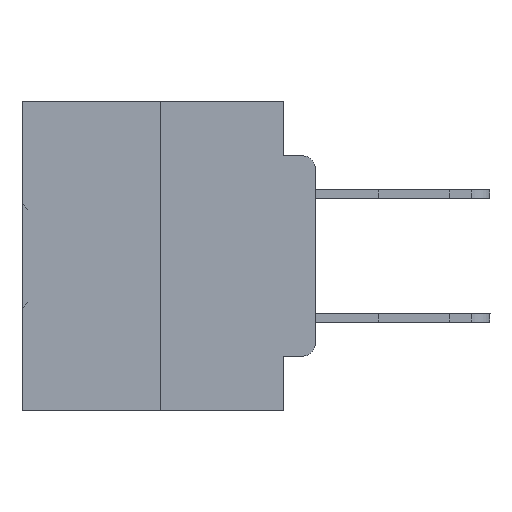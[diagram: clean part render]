
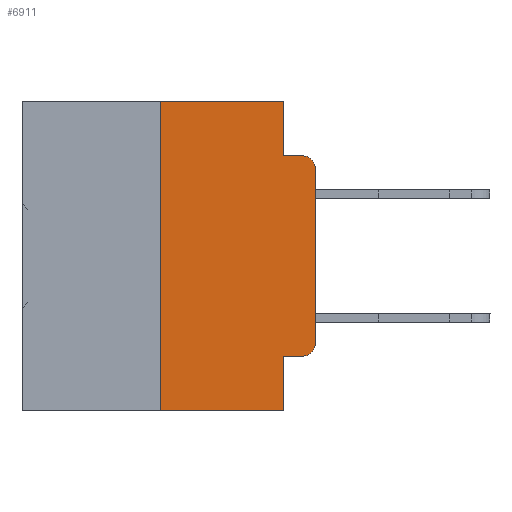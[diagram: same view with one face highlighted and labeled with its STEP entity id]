
A CAD part, left-side view. The second image highlights one B-rep face of the part: STEP entity #6911.
In plain terms, the highlighted planar face has unit normal (-1, 0, 0).
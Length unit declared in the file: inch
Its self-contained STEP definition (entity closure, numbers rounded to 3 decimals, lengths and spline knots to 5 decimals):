
#1112 = EDGE_CURVE ( 'NONE', #8492, #10037, #37181, .T. ) ;
#1606 = DIRECTION ( 'NONE',  ( 0., -1., 0. ) ) ;
#2533 = VECTOR ( 'NONE', #21552, 39.37008 ) ;
#2599 = CARTESIAN_POINT ( 'NONE',  ( 0., 0.051, -0.0885 ) ) ;
#3186 = DIRECTION ( 'NONE',  ( 0., 0., -1. ) ) ;
#3960 = EDGE_LOOP ( 'NONE', ( #23107, #32588, #10582, #7675, #37081, #15077, #35755, #18304, #5383, #36278 ) ) ;
#5097 = LINE ( 'NONE', #10026, #2533 ) ;
#5383 = ORIENTED_EDGE ( 'NONE', *, *, #35285, .T. ) ;
#5484 = DIRECTION ( 'NONE',  ( 0., 0., -1. ) ) ;
#6058 = AXIS2_PLACEMENT_3D ( 'NONE', #34213, #8325, #31364 ) ;
#6208 = VECTOR ( 'NONE', #13456, 39.37008 ) ;
#6746 = AXIS2_PLACEMENT_3D ( 'NONE', #25912, #11363, #5484 ) ;
#6911 = ADVANCED_FACE ( 'NONE', ( #29285 ), #20406, .F. ) ;
#6920 = VERTEX_POINT ( 'NONE', #20225 ) ;
#6921 = EDGE_CURVE ( 'NONE', #34505, #21723, #31728, .T. ) ;
#7185 = VECTOR ( 'NONE', #19292, 39.37008 ) ;
#7336 = VECTOR ( 'NONE', #23421, 39.37008 ) ;
#7675 = ORIENTED_EDGE ( 'NONE', *, *, #26882, .F. ) ;
#7763 = CARTESIAN_POINT ( 'NONE',  ( 0., 0.051, 0. ) ) ;
#7807 = DIRECTION ( 'NONE',  ( 0., -1., 0. ) ) ;
#8325 = DIRECTION ( 'NONE',  ( 1., 0., 0. ) ) ;
#8492 = VERTEX_POINT ( 'NONE', #13720 ) ;
#8664 = CARTESIAN_POINT ( 'NONE',  ( 0., 0.051, -0.5 ) ) ;
#9150 = CIRCLE ( 'NONE', #6746, 0.02 ) ;
#10026 = CARTESIAN_POINT ( 'NONE',  ( 0., 0.473, -0.5 ) ) ;
#10037 = VERTEX_POINT ( 'NONE', #33516 ) ;
#10467 = CARTESIAN_POINT ( 'NONE',  ( 0., 0., -0.3915 ) ) ;
#10582 = ORIENTED_EDGE ( 'NONE', *, *, #1112, .F. ) ;
#11300 = VECTOR ( 'NONE', #1606, 39.37008 ) ;
#11363 = DIRECTION ( 'NONE',  ( -1., 0., 0. ) ) ;
#11385 = EDGE_CURVE ( 'NONE', #6920, #34505, #27099, .T. ) ;
#11714 = CARTESIAN_POINT ( 'NONE',  ( 0., 0.02, -0.3915 ) ) ;
#11737 = LINE ( 'NONE', #23240, #7336 ) ;
#13456 = DIRECTION ( 'NONE',  ( 0., 0., 1. ) ) ;
#13720 = CARTESIAN_POINT ( 'NONE',  ( 0., 0.051, -0.0885 ) ) ;
#13979 = EDGE_CURVE ( 'NONE', #21723, #10037, #9150, .T. ) ;
#14080 = EDGE_CURVE ( 'NONE', #36725, #35102, #11737, .T. ) ;
#14435 = AXIS2_PLACEMENT_3D ( 'NONE', #11714, #34726, #3186 ) ;
#15077 = ORIENTED_EDGE ( 'NONE', *, *, #15186, .F. ) ;
#15186 = EDGE_CURVE ( 'NONE', #33702, #35637, #19485, .T. ) ;
#15306 = CARTESIAN_POINT ( 'NONE',  ( 0., 0., 0. ) ) ;
#15616 = CARTESIAN_POINT ( 'NONE',  ( 0., 0.051, -0.4115 ) ) ;
#16781 = DIRECTION ( 'NONE',  ( 0., -1., 0. ) ) ;
#17046 = CARTESIAN_POINT ( 'NONE',  ( 0., 0.25, 0. ) ) ;
#18291 = VERTEX_POINT ( 'NONE', #25071 ) ;
#18304 = ORIENTED_EDGE ( 'NONE', *, *, #14080, .F. ) ;
#19292 = DIRECTION ( 'NONE',  ( 0., 0., -1. ) ) ;
#19485 = LINE ( 'NONE', #17046, #6208 ) ;
#19522 = CARTESIAN_POINT ( 'NONE',  ( 0., 0.473, 0. ) ) ;
#20225 = CARTESIAN_POINT ( 'NONE',  ( 0., 0.02, -0.4115 ) ) ;
#20406 = PLANE ( 'NONE',  #6058 ) ;
#21552 = DIRECTION ( 'NONE',  ( 0., -1., 0. ) ) ;
#21723 = VERTEX_POINT ( 'NONE', #35341 ) ;
#21993 = LINE ( 'NONE', #19522, #24067 ) ;
#23107 = ORIENTED_EDGE ( 'NONE', *, *, #6921, .T. ) ;
#23240 = CARTESIAN_POINT ( 'NONE',  ( 0., 0.051, 0. ) ) ;
#23421 = DIRECTION ( 'NONE',  ( 0., 0., -1. ) ) ;
#24067 = VECTOR ( 'NONE', #7807, 39.37008 ) ;
#24327 = LINE ( 'NONE', #15616, #11300 ) ;
#25071 = CARTESIAN_POINT ( 'NONE',  ( 0., 0.051, 0. ) ) ;
#25854 = CARTESIAN_POINT ( 'NONE',  ( 0., 0.25, -0.5 ) ) ;
#25912 = CARTESIAN_POINT ( 'NONE',  ( 0., 0.02, -0.1085 ) ) ;
#26406 = EDGE_CURVE ( 'NONE', #35637, #18291, #21993, .T. ) ;
#26882 = EDGE_CURVE ( 'NONE', #18291, #8492, #33646, .T. ) ;
#27099 = CIRCLE ( 'NONE', #14435, 0.02 ) ;
#29285 = FACE_OUTER_BOUND ( 'NONE', #3960, .T. ) ;
#29839 = CARTESIAN_POINT ( 'NONE',  ( 0., 0.051, -0.4115 ) ) ;
#30779 = VECTOR ( 'NONE', #32856, 39.37008 ) ;
#31364 = DIRECTION ( 'NONE',  ( 0., 0., -1. ) ) ;
#31728 = LINE ( 'NONE', #15306, #30779 ) ;
#32420 = VECTOR ( 'NONE', #16781, 39.37008 ) ;
#32588 = ORIENTED_EDGE ( 'NONE', *, *, #13979, .T. ) ;
#32856 = DIRECTION ( 'NONE',  ( 0., 0., 1. ) ) ;
#33151 = EDGE_CURVE ( 'NONE', #33702, #35102, #5097, .T. ) ;
#33516 = CARTESIAN_POINT ( 'NONE',  ( 0., 0.02, -0.0885 ) ) ;
#33646 = LINE ( 'NONE', #7763, #7185 ) ;
#33702 = VERTEX_POINT ( 'NONE', #25854 ) ;
#34213 = CARTESIAN_POINT ( 'NONE',  ( 0., 0.473, 0. ) ) ;
#34505 = VERTEX_POINT ( 'NONE', #10467 ) ;
#34726 = DIRECTION ( 'NONE',  ( -1., 0., 0. ) ) ;
#34840 = CARTESIAN_POINT ( 'NONE',  ( 0., 0.25, 0. ) ) ;
#35102 = VERTEX_POINT ( 'NONE', #8664 ) ;
#35285 = EDGE_CURVE ( 'NONE', #36725, #6920, #24327, .T. ) ;
#35341 = CARTESIAN_POINT ( 'NONE',  ( 0., 0., -0.1085 ) ) ;
#35637 = VERTEX_POINT ( 'NONE', #34840 ) ;
#35755 = ORIENTED_EDGE ( 'NONE', *, *, #33151, .T. ) ;
#36278 = ORIENTED_EDGE ( 'NONE', *, *, #11385, .T. ) ;
#36725 = VERTEX_POINT ( 'NONE', #29839 ) ;
#37081 = ORIENTED_EDGE ( 'NONE', *, *, #26406, .F. ) ;
#37181 = LINE ( 'NONE', #2599, #32420 ) ;
